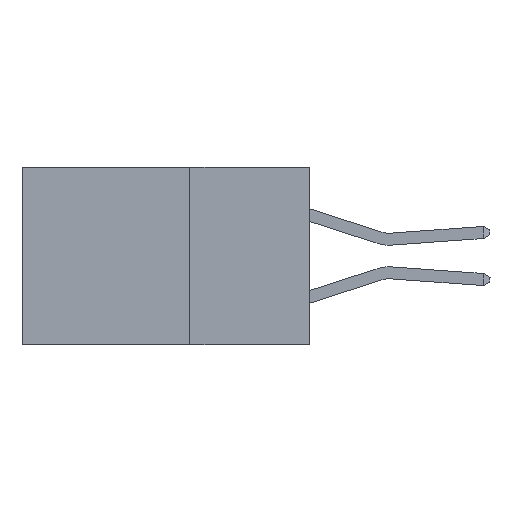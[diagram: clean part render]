
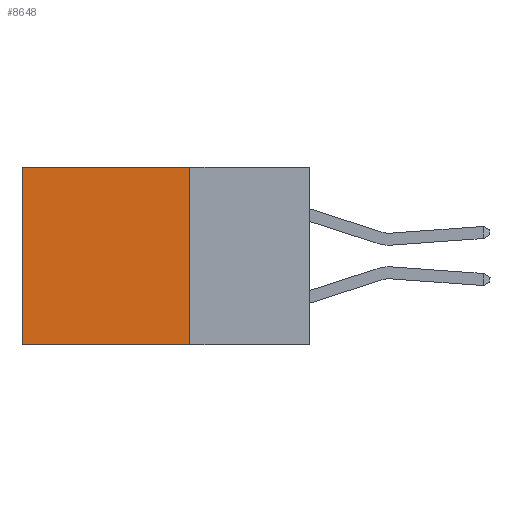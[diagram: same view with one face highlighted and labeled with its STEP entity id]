
A CAD part, left-side view. The second image highlights one B-rep face of the part: STEP entity #8648.
In plain terms, the highlighted planar face has unit normal (-1, 0, 0).
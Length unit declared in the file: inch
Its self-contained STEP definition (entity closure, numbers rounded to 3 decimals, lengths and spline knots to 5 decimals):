
#71 = CARTESIAN_POINT ( 'NONE',  ( 0.2615, 0.25, 0. ) ) ;
#287 = CARTESIAN_POINT ( 'NONE',  ( 0.2615, 0.25, -0.37 ) ) ;
#964 = LINE ( 'NONE', #2322, #2694 ) ;
#1719 = VECTOR ( 'NONE', #3142, 39.37008 ) ;
#1836 = LINE ( 'NONE', #287, #3822 ) ;
#2237 = VERTEX_POINT ( 'NONE', #5415 ) ;
#2322 = CARTESIAN_POINT ( 'NONE',  ( 0.2615, 0.25, -0.37 ) ) ;
#2334 = VECTOR ( 'NONE', #7470, 39.37008 ) ;
#2694 = VECTOR ( 'NONE', #9321, 39.37008 ) ;
#2712 = DIRECTION ( 'NONE',  ( 0., 0., -1. ) ) ;
#2721 = VERTEX_POINT ( 'NONE', #3124 ) ;
#3017 = CARTESIAN_POINT ( 'NONE',  ( 0.2615, 0.25, -0.37 ) ) ;
#3124 = CARTESIAN_POINT ( 'NONE',  ( 0.2615, 0.6, 0. ) ) ;
#3142 = DIRECTION ( 'NONE',  ( 0., 0., -1. ) ) ;
#3681 = ORIENTED_EDGE ( 'NONE', *, *, #3973, .F. ) ;
#3757 = DIRECTION ( 'NONE',  ( 1., 0., 0. ) ) ;
#3822 = VECTOR ( 'NONE', #2712, 39.37008 ) ;
#3826 = LINE ( 'NONE', #3872, #1719 ) ;
#3872 = CARTESIAN_POINT ( 'NONE',  ( 0.2615, 0.6, -0.37 ) ) ;
#3973 = EDGE_CURVE ( 'NONE', #8544, #6000, #1836, .T. ) ;
#4441 = LINE ( 'NONE', #5126, #2334 ) ;
#4593 = EDGE_LOOP ( 'NONE', ( #5769, #5569, #3681, #8577 ) ) ;
#5126 = CARTESIAN_POINT ( 'NONE',  ( 0.2615, 0.25, 0. ) ) ;
#5395 = FACE_OUTER_BOUND ( 'NONE', #4593, .T. ) ;
#5415 = CARTESIAN_POINT ( 'NONE',  ( 0.2615, 0.6, -0.37 ) ) ;
#5569 = ORIENTED_EDGE ( 'NONE', *, *, #8688, .F. ) ;
#5769 = ORIENTED_EDGE ( 'NONE', *, *, #9110, .T. ) ;
#5843 = AXIS2_PLACEMENT_3D ( 'NONE', #3017, #3757, #8461 ) ;
#6000 = VERTEX_POINT ( 'NONE', #7566 ) ;
#7470 = DIRECTION ( 'NONE',  ( 0., 1., 0. ) ) ;
#7566 = CARTESIAN_POINT ( 'NONE',  ( 0.2615, 0.25, -0.37 ) ) ;
#7765 = EDGE_CURVE ( 'NONE', #8544, #2721, #4441, .T. ) ;
#8461 = DIRECTION ( 'NONE',  ( 0., 0., -1. ) ) ;
#8544 = VERTEX_POINT ( 'NONE', #71 ) ;
#8577 = ORIENTED_EDGE ( 'NONE', *, *, #7765, .T. ) ;
#8648 = ADVANCED_FACE ( 'NONE', ( #5395 ), #10052, .F. ) ;
#8688 = EDGE_CURVE ( 'NONE', #6000, #2237, #964, .T. ) ;
#9110 = EDGE_CURVE ( 'NONE', #2721, #2237, #3826, .T. ) ;
#9321 = DIRECTION ( 'NONE',  ( 0., 1., 0. ) ) ;
#10052 = PLANE ( 'NONE',  #5843 ) ;
